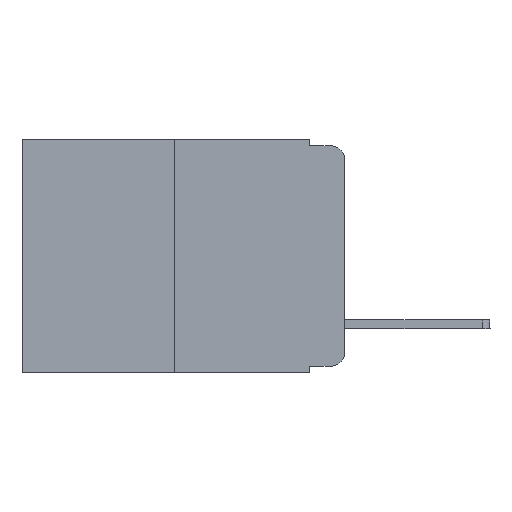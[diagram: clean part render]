
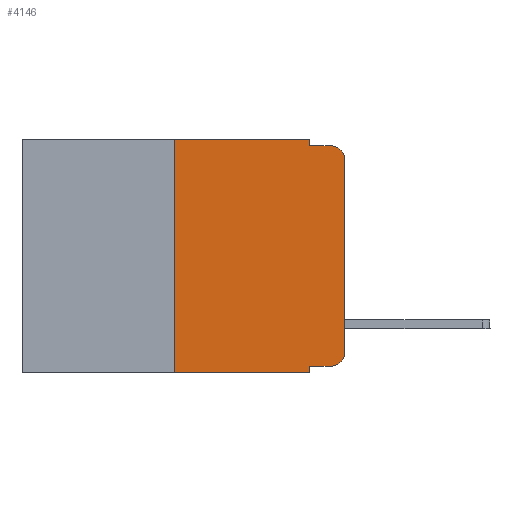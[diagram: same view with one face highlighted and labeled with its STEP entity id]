
A CAD part, left-side view. The second image highlights one B-rep face of the part: STEP entity #4146.
In plain terms, the highlighted planar face has unit normal (-1, 0, 0).
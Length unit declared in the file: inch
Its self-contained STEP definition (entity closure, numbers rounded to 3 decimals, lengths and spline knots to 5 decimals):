
#25 = VERTEX_POINT ( 'NONE', #14208 ) ;
#511 = LINE ( 'NONE', #10935, #11920 ) ;
#524 = ORIENTED_EDGE ( 'NONE', *, *, #1216, .T. ) ;
#543 = DIRECTION ( 'NONE',  ( -1., 0., 0. ) ) ;
#1216 = EDGE_CURVE ( 'NONE', #11229, #2682, #15335, .T. ) ;
#1283 = CARTESIAN_POINT ( 'NONE',  ( 0., 0.051, -0.333 ) ) ;
#1306 = VERTEX_POINT ( 'NONE', #8837 ) ;
#1461 = CIRCLE ( 'NONE', #16035, 0.02 ) ;
#1911 = VERTEX_POINT ( 'NONE', #12154 ) ;
#1988 = ORIENTED_EDGE ( 'NONE', *, *, #15010, .F. ) ;
#2009 = CARTESIAN_POINT ( 'NONE',  ( 0., 0.02, -0.313 ) ) ;
#2385 = ORIENTED_EDGE ( 'NONE', *, *, #6647, .F. ) ;
#2486 = VERTEX_POINT ( 'NONE', #8231 ) ;
#2591 = EDGE_CURVE ( 'NONE', #25, #5223, #15934, .T. ) ;
#2641 = ORIENTED_EDGE ( 'NONE', *, *, #15213, .F. ) ;
#2682 = VERTEX_POINT ( 'NONE', #6267 ) ;
#2919 = ORIENTED_EDGE ( 'NONE', *, *, #7953, .F. ) ;
#3160 = CARTESIAN_POINT ( 'NONE',  ( 0., 0.25, 0. ) ) ;
#3703 = DIRECTION ( 'NONE',  ( 0., 0., -1. ) ) ;
#4146 = ADVANCED_FACE ( 'NONE', ( #6491 ), #14112, .F. ) ;
#4384 = VERTEX_POINT ( 'NONE', #13365 ) ;
#4863 = CARTESIAN_POINT ( 'NONE',  ( 0., 0.051, -0.01 ) ) ;
#5223 = VERTEX_POINT ( 'NONE', #7692 ) ;
#5614 = ORIENTED_EDGE ( 'NONE', *, *, #7056, .T. ) ;
#5742 = DIRECTION ( 'NONE',  ( 0., -1., 0. ) ) ;
#5807 = LINE ( 'NONE', #9947, #15575 ) ;
#5947 = DIRECTION ( 'NONE',  ( 0., 0., -1. ) ) ;
#6262 = EDGE_CURVE ( 'NONE', #10883, #11229, #5807, .T. ) ;
#6267 = CARTESIAN_POINT ( 'NONE',  ( 0., 0.02, -0.01 ) ) ;
#6460 = LINE ( 'NONE', #13584, #9037 ) ;
#6491 = FACE_OUTER_BOUND ( 'NONE', #7689, .T. ) ;
#6647 = EDGE_CURVE ( 'NONE', #1306, #1911, #13779, .T. ) ;
#7056 = EDGE_CURVE ( 'NONE', #1306, #15682, #13141, .T. ) ;
#7079 = CARTESIAN_POINT ( 'NONE',  ( 0., 0., -0.313 ) ) ;
#7346 = CARTESIAN_POINT ( 'NONE',  ( 0., 0.473, 0. ) ) ;
#7624 = ORIENTED_EDGE ( 'NONE', *, *, #6262, .T. ) ;
#7689 = EDGE_LOOP ( 'NONE', ( #7624, #524, #2919, #11723, #2641, #1988, #11670, #2385, #5614, #10688 ) ) ;
#7692 = CARTESIAN_POINT ( 'NONE',  ( 0., 0.051, -0.01 ) ) ;
#7833 = EDGE_CURVE ( 'NONE', #15682, #10883, #1461, .T. ) ;
#7847 = LINE ( 'NONE', #3160, #11436 ) ;
#7953 = EDGE_CURVE ( 'NONE', #5223, #2682, #8305, .T. ) ;
#8018 = DIRECTION ( 'NONE',  ( 0., 0., -1. ) ) ;
#8231 = CARTESIAN_POINT ( 'NONE',  ( 0., 0.25, 0. ) ) ;
#8305 = LINE ( 'NONE', #4863, #11883 ) ;
#8562 = CARTESIAN_POINT ( 'NONE',  ( 0., 0., -0.03 ) ) ;
#8837 = CARTESIAN_POINT ( 'NONE',  ( 0., 0.051, -0.333 ) ) ;
#8973 = VECTOR ( 'NONE', #8018, 39.37008 ) ;
#9037 = VECTOR ( 'NONE', #12241, 39.37008 ) ;
#9141 = VECTOR ( 'NONE', #5947, 39.37008 ) ;
#9947 = CARTESIAN_POINT ( 'NONE',  ( 0., 0., 0. ) ) ;
#10105 = AXIS2_PLACEMENT_3D ( 'NONE', #7346, #16132, #3703 ) ;
#10688 = ORIENTED_EDGE ( 'NONE', *, *, #7833, .T. ) ;
#10883 = VERTEX_POINT ( 'NONE', #7079 ) ;
#10935 = CARTESIAN_POINT ( 'NONE',  ( 0., 0.473, -0.343 ) ) ;
#11229 = VERTEX_POINT ( 'NONE', #8562 ) ;
#11436 = VECTOR ( 'NONE', #13455, 39.37008 ) ;
#11670 = ORIENTED_EDGE ( 'NONE', *, *, #13100, .T. ) ;
#11723 = ORIENTED_EDGE ( 'NONE', *, *, #2591, .F. ) ;
#11883 = VECTOR ( 'NONE', #16160, 39.37008 ) ;
#11920 = VECTOR ( 'NONE', #5742, 39.37008 ) ;
#12120 = DIRECTION ( 'NONE',  ( 0., 0., -1. ) ) ;
#12154 = CARTESIAN_POINT ( 'NONE',  ( 0., 0.051, -0.343 ) ) ;
#12241 = DIRECTION ( 'NONE',  ( 0., -1., 0. ) ) ;
#12345 = DIRECTION ( 'NONE',  ( 0., 0., 1. ) ) ;
#12363 = CARTESIAN_POINT ( 'NONE',  ( 0., 0.051, 0. ) ) ;
#12527 = AXIS2_PLACEMENT_3D ( 'NONE', #15126, #13906, #15276 ) ;
#13100 = EDGE_CURVE ( 'NONE', #4384, #1911, #511, .T. ) ;
#13141 = LINE ( 'NONE', #1283, #16188 ) ;
#13365 = CARTESIAN_POINT ( 'NONE',  ( 0., 0.25, -0.343 ) ) ;
#13455 = DIRECTION ( 'NONE',  ( 0., 0., 1. ) ) ;
#13584 = CARTESIAN_POINT ( 'NONE',  ( 0., 0.473, 0. ) ) ;
#13609 = CARTESIAN_POINT ( 'NONE',  ( 0., 0.02, -0.333 ) ) ;
#13779 = LINE ( 'NONE', #15533, #8973 ) ;
#13906 = DIRECTION ( 'NONE',  ( -1., 0., 0. ) ) ;
#14112 = PLANE ( 'NONE',  #10105 ) ;
#14171 = DIRECTION ( 'NONE',  ( 0., -1., 0. ) ) ;
#14208 = CARTESIAN_POINT ( 'NONE',  ( 0., 0.051, 0. ) ) ;
#15010 = EDGE_CURVE ( 'NONE', #4384, #2486, #7847, .T. ) ;
#15126 = CARTESIAN_POINT ( 'NONE',  ( 0., 0.02, -0.03 ) ) ;
#15213 = EDGE_CURVE ( 'NONE', #2486, #25, #6460, .T. ) ;
#15276 = DIRECTION ( 'NONE',  ( 0., 0., -1. ) ) ;
#15335 = CIRCLE ( 'NONE', #12527, 0.02 ) ;
#15533 = CARTESIAN_POINT ( 'NONE',  ( 0., 0.051, 0. ) ) ;
#15575 = VECTOR ( 'NONE', #12345, 39.37008 ) ;
#15682 = VERTEX_POINT ( 'NONE', #13609 ) ;
#15934 = LINE ( 'NONE', #12363, #9141 ) ;
#16035 = AXIS2_PLACEMENT_3D ( 'NONE', #2009, #543, #12120 ) ;
#16132 = DIRECTION ( 'NONE',  ( 1., 0., 0. ) ) ;
#16160 = DIRECTION ( 'NONE',  ( 0., -1., 0. ) ) ;
#16188 = VECTOR ( 'NONE', #14171, 39.37008 ) ;
